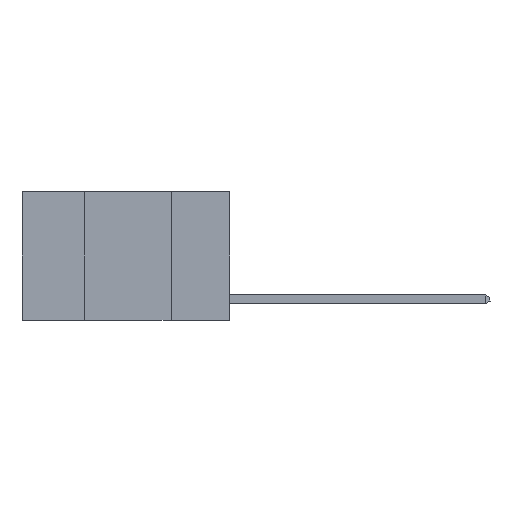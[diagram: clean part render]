
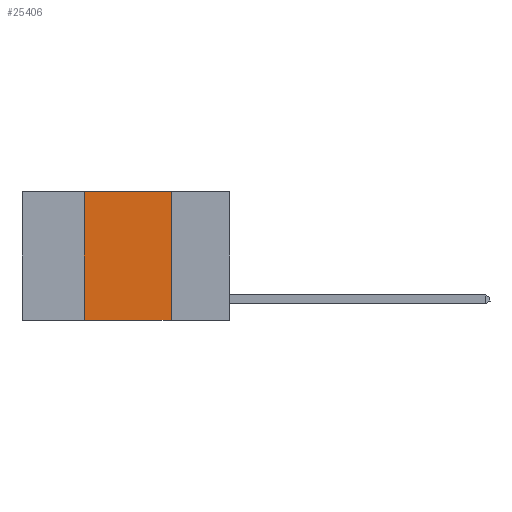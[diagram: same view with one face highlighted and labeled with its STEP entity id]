
A CAD part, left-side view. The second image highlights one B-rep face of the part: STEP entity #25406.
In plain terms, the highlighted planar face has unit normal (-1, 0, 0).
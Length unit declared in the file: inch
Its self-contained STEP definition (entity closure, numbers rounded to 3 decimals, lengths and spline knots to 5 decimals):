
#61 = CARTESIAN_POINT ( 'NONE',  ( 0., 0.42, -0.37 ) ) ;
#225 = VECTOR ( 'NONE', #13830, 39.37008 ) ;
#467 = VECTOR ( 'NONE', #4870, 39.37008 ) ;
#527 = ORIENTED_EDGE ( 'NONE', *, *, #22828, .F. ) ;
#967 = ORIENTED_EDGE ( 'NONE', *, *, #6466, .F. ) ;
#1813 = VERTEX_POINT ( 'NONE', #61 ) ;
#1929 = DIRECTION ( 'NONE',  ( 1., 0., 0. ) ) ;
#2621 = CARTESIAN_POINT ( 'NONE',  ( 0., 0.42, 0. ) ) ;
#2669 = VERTEX_POINT ( 'NONE', #17105 ) ;
#2922 = LINE ( 'NONE', #9623, #467 ) ;
#4002 = VECTOR ( 'NONE', #24490, 39.37008 ) ;
#4870 = DIRECTION ( 'NONE',  ( 0., -1., 0. ) ) ;
#4914 = VERTEX_POINT ( 'NONE', #13783 ) ;
#5477 = CARTESIAN_POINT ( 'NONE',  ( 0., 0.6, 0. ) ) ;
#6466 = EDGE_CURVE ( 'NONE', #2669, #14332, #23531, .T. ) ;
#8542 = LINE ( 'NONE', #5477, #19182 ) ;
#9623 = CARTESIAN_POINT ( 'NONE',  ( 0., 0.6, -0.37 ) ) ;
#10464 = EDGE_CURVE ( 'NONE', #1813, #14332, #2922, .T. ) ;
#10840 = CARTESIAN_POINT ( 'NONE',  ( 0., 0.6, 0. ) ) ;
#10986 = CARTESIAN_POINT ( 'NONE',  ( 0., 0.17, 0. ) ) ;
#11042 = DIRECTION ( 'NONE',  ( 0., 0., -1. ) ) ;
#12113 = DIRECTION ( 'NONE',  ( 0., -1., 0. ) ) ;
#12375 = FACE_OUTER_BOUND ( 'NONE', #19656, .T. ) ;
#12914 = ORIENTED_EDGE ( 'NONE', *, *, #18876, .F. ) ;
#13783 = CARTESIAN_POINT ( 'NONE',  ( 0., 0.42, 0. ) ) ;
#13830 = DIRECTION ( 'NONE',  ( 0., 0., 1. ) ) ;
#14332 = VERTEX_POINT ( 'NONE', #14478 ) ;
#14431 = ORIENTED_EDGE ( 'NONE', *, *, #10464, .T. ) ;
#14478 = CARTESIAN_POINT ( 'NONE',  ( 0., 0.17, -0.37 ) ) ;
#17105 = CARTESIAN_POINT ( 'NONE',  ( 0., 0.17, 0. ) ) ;
#18298 = LINE ( 'NONE', #2621, #225 ) ;
#18876 = EDGE_CURVE ( 'NONE', #1813, #4914, #18298, .T. ) ;
#19182 = VECTOR ( 'NONE', #12113, 39.37008 ) ;
#19656 = EDGE_LOOP ( 'NONE', ( #967, #527, #12914, #14431 ) ) ;
#22554 = PLANE ( 'NONE',  #27754 ) ;
#22828 = EDGE_CURVE ( 'NONE', #4914, #2669, #8542, .T. ) ;
#23531 = LINE ( 'NONE', #10986, #4002 ) ;
#24490 = DIRECTION ( 'NONE',  ( 0., 0., -1. ) ) ;
#25406 = ADVANCED_FACE ( 'NONE', ( #12375 ), #22554, .F. ) ;
#27754 = AXIS2_PLACEMENT_3D ( 'NONE', #10840, #1929, #11042 ) ;
